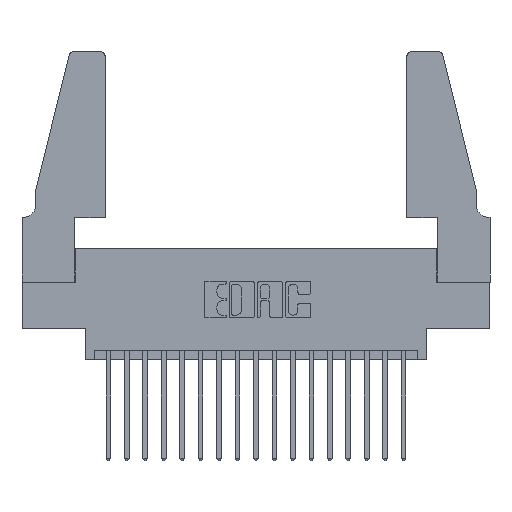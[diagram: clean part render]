
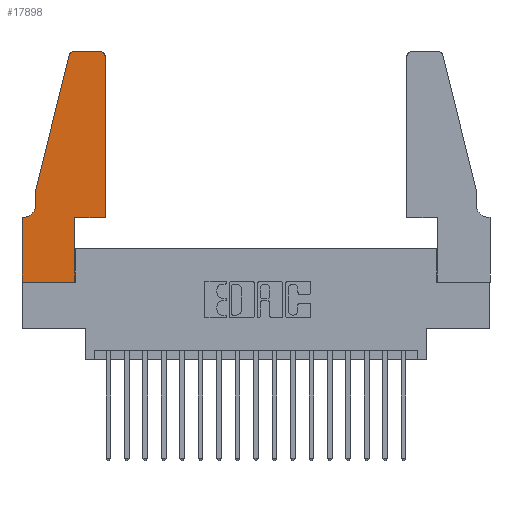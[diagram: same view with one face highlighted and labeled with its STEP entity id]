
A CAD part, top view. The second image highlights one B-rep face of the part: STEP entity #17898.
In plain terms, the highlighted planar face has unit normal (0, 0, 1).
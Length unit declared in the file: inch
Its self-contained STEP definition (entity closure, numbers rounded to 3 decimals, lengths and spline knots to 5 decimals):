
#21 = LINE ( 'NONE', #6034, #14858 ) ;
#507 = CARTESIAN_POINT ( 'NONE',  ( 0., 0., 0.37 ) ) ;
#840 = VERTEX_POINT ( 'NONE', #17186 ) ;
#1100 = DIRECTION ( 'NONE',  ( 0., 0., 1. ) ) ;
#1206 = DIRECTION ( 'NONE',  ( 0., 0., 1. ) ) ;
#1259 = ORIENTED_EDGE ( 'NONE', *, *, #5324, .T. ) ;
#1318 = CIRCLE ( 'NONE', #5021, 0.03 ) ;
#1538 = VECTOR ( 'NONE', #3519, 39.37008 ) ;
#1597 = VECTOR ( 'NONE', #3736, 39.37008 ) ;
#1655 = CARTESIAN_POINT ( 'NONE',  ( 0.4505, 0.35, 0.37 ) ) ;
#1902 = EDGE_CURVE ( 'NONE', #840, #3299, #11785, .T. ) ;
#2050 = EDGE_CURVE ( 'NONE', #11786, #7274, #18245, .T. ) ;
#2129 = CARTESIAN_POINT ( 'NONE',  ( 0.0055, 0.35, 0.37 ) ) ;
#2143 = EDGE_CURVE ( 'NONE', #5489, #8477, #16881, .T. ) ;
#2196 = ORIENTED_EDGE ( 'NONE', *, *, #7530, .T. ) ;
#2276 = CARTESIAN_POINT ( 'NONE',  ( 0.4505, 0.35, 0.37 ) ) ;
#2293 = FACE_OUTER_BOUND ( 'NONE', #11390, .T. ) ;
#3299 = VERTEX_POINT ( 'NONE', #5409 ) ;
#3519 = DIRECTION ( 'NONE',  ( 1., 0., 0. ) ) ;
#3605 = VERTEX_POINT ( 'NONE', #13110 ) ;
#3736 = DIRECTION ( 'NONE',  ( 0., 1., 0. ) ) ;
#3822 = CARTESIAN_POINT ( 'NONE',  ( 0.2865, 0.35, 0.37 ) ) ;
#3868 = VECTOR ( 'NONE', #7863, 39.37008 ) ;
#3891 = CARTESIAN_POINT ( 'NONE',  ( 0.4205, 1.25, 0.37 ) ) ;
#3926 = LINE ( 'NONE', #3822, #7421 ) ;
#4071 = VERTEX_POINT ( 'NONE', #13634 ) ;
#4606 = AXIS2_PLACEMENT_3D ( 'NONE', #5490, #1100, #11475 ) ;
#5021 = AXIS2_PLACEMENT_3D ( 'NONE', #5882, #16181, #7387 ) ;
#5324 = EDGE_CURVE ( 'NONE', #3299, #8935, #12471, .T. ) ;
#5409 = CARTESIAN_POINT ( 'NONE',  ( 0., 0., 0.37 ) ) ;
#5489 = VERTEX_POINT ( 'NONE', #3891 ) ;
#5490 = CARTESIAN_POINT ( 'NONE',  ( 0., 0.35, 0.37 ) ) ;
#5882 = CARTESIAN_POINT ( 'NONE',  ( 0.284, 1.22, 0.37 ) ) ;
#6034 = CARTESIAN_POINT ( 'NONE',  ( 0.0755, 0.5, 0.37 ) ) ;
#6742 = CARTESIAN_POINT ( 'NONE',  ( 0.4505, 0.35, 0.37 ) ) ;
#7274 = VERTEX_POINT ( 'NONE', #2129 ) ;
#7327 = DIRECTION ( 'NONE',  ( 0., -1., 0. ) ) ;
#7387 = DIRECTION ( 'NONE',  ( 1., 0., 0. ) ) ;
#7421 = VECTOR ( 'NONE', #9818, 39.37008 ) ;
#7530 = EDGE_CURVE ( 'NONE', #4071, #5489, #17375, .T. ) ;
#7652 = EDGE_CURVE ( 'NONE', #7274, #840, #15588, .T. ) ;
#7863 = DIRECTION ( 'NONE',  ( -0.239, -0.971, 0. ) ) ;
#7945 = AXIS2_PLACEMENT_3D ( 'NONE', #10101, #1206, #11587 ) ;
#8123 = CARTESIAN_POINT ( 'NONE',  ( 0.2865, 0.35, 0.37 ) ) ;
#8232 = VECTOR ( 'NONE', #10280, 39.37008 ) ;
#8409 = VERTEX_POINT ( 'NONE', #10510 ) ;
#8477 = VERTEX_POINT ( 'NONE', #13635 ) ;
#8532 = EDGE_CURVE ( 'NONE', #8409, #3605, #11319, .T. ) ;
#8621 = ORIENTED_EDGE ( 'NONE', *, *, #17179, .T. ) ;
#8866 = EDGE_CURVE ( 'NONE', #8477, #8409, #1318, .T. ) ;
#8911 = LINE ( 'NONE', #1655, #12887 ) ;
#8935 = VERTEX_POINT ( 'NONE', #14876 ) ;
#9498 = ORIENTED_EDGE ( 'NONE', *, *, #7652, .T. ) ;
#9517 = LINE ( 'NONE', #2276, #1597 ) ;
#9774 = CARTESIAN_POINT ( 'NONE',  ( 0.0055, 0.42, 0.37 ) ) ;
#9818 = DIRECTION ( 'NONE',  ( 0., 1., 0. ) ) ;
#9977 = AXIS2_PLACEMENT_3D ( 'NONE', #9774, #11076, #11170 ) ;
#9987 = PLANE ( 'NONE',  #4606 ) ;
#10101 = CARTESIAN_POINT ( 'NONE',  ( 0.4205, 1.22, 0.37 ) ) ;
#10129 = ORIENTED_EDGE ( 'NONE', *, *, #11989, .T. ) ;
#10280 = DIRECTION ( 'NONE',  ( -1., 0., 0. ) ) ;
#10510 = CARTESIAN_POINT ( 'NONE',  ( 0.25487, 1.22718, 0.37 ) ) ;
#11076 = DIRECTION ( 'NONE',  ( 0., 0., -1. ) ) ;
#11170 = DIRECTION ( 'NONE',  ( -1., 0., 0. ) ) ;
#11319 = LINE ( 'NONE', #18081, #3868 ) ;
#11334 = VECTOR ( 'NONE', #7327, 39.37008 ) ;
#11390 = EDGE_LOOP ( 'NONE', ( #13086, #13402, #16027, #10129, #18684, #9498, #16604, #1259, #8621, #15460, #16996, #2196 ) ) ;
#11475 = DIRECTION ( 'NONE',  ( 1., 0., 0. ) ) ;
#11587 = DIRECTION ( 'NONE',  ( 1., 0., 0. ) ) ;
#11785 = LINE ( 'NONE', #507, #11334 ) ;
#11786 = VERTEX_POINT ( 'NONE', #18594 ) ;
#11989 = EDGE_CURVE ( 'NONE', #3605, #11786, #21, .T. ) ;
#12042 = DIRECTION ( 'NONE',  ( 1., 0., 0. ) ) ;
#12471 = LINE ( 'NONE', #13910, #1538 ) ;
#12887 = VECTOR ( 'NONE', #12042, 39.37008 ) ;
#13086 = ORIENTED_EDGE ( 'NONE', *, *, #2143, .T. ) ;
#13110 = CARTESIAN_POINT ( 'NONE',  ( 0.0755, 0.5, 0.37 ) ) ;
#13402 = ORIENTED_EDGE ( 'NONE', *, *, #8866, .T. ) ;
#13634 = CARTESIAN_POINT ( 'NONE',  ( 0.4505, 1.22, 0.37 ) ) ;
#13635 = CARTESIAN_POINT ( 'NONE',  ( 0.284, 1.25, 0.37 ) ) ;
#13910 = CARTESIAN_POINT ( 'NONE',  ( 0., 0., 0.37 ) ) ;
#14063 = VERTEX_POINT ( 'NONE', #8123 ) ;
#14094 = EDGE_CURVE ( 'NONE', #14117, #4071, #9517, .T. ) ;
#14117 = VERTEX_POINT ( 'NONE', #6742 ) ;
#14733 = CARTESIAN_POINT ( 'NONE',  ( 0.0755, 0.35, 0.37 ) ) ;
#14858 = VECTOR ( 'NONE', #16390, 39.37008 ) ;
#14876 = CARTESIAN_POINT ( 'NONE',  ( 0.2865, 0., 0.37 ) ) ;
#14994 = EDGE_CURVE ( 'NONE', #14063, #14117, #8911, .T. ) ;
#15460 = ORIENTED_EDGE ( 'NONE', *, *, #14994, .T. ) ;
#15588 = LINE ( 'NONE', #14733, #8232 ) ;
#15710 = DIRECTION ( 'NONE',  ( -1., 0., 0. ) ) ;
#16027 = ORIENTED_EDGE ( 'NONE', *, *, #8532, .T. ) ;
#16181 = DIRECTION ( 'NONE',  ( 0., 0., 1. ) ) ;
#16390 = DIRECTION ( 'NONE',  ( 0., -1., 0. ) ) ;
#16431 = VECTOR ( 'NONE', #15710, 39.37008 ) ;
#16604 = ORIENTED_EDGE ( 'NONE', *, *, #1902, .T. ) ;
#16881 = LINE ( 'NONE', #17586, #16431 ) ;
#16996 = ORIENTED_EDGE ( 'NONE', *, *, #14094, .T. ) ;
#17179 = EDGE_CURVE ( 'NONE', #8935, #14063, #3926, .T. ) ;
#17186 = CARTESIAN_POINT ( 'NONE',  ( 0., 0.35, 0.37 ) ) ;
#17375 = CIRCLE ( 'NONE', #7945, 0.03 ) ;
#17586 = CARTESIAN_POINT ( 'NONE',  ( 0.2605, 1.25, 0.37 ) ) ;
#17898 = ADVANCED_FACE ( 'NONE', ( #2293 ), #9987, .T. ) ;
#18081 = CARTESIAN_POINT ( 'NONE',  ( 0.0755, 0.5, 0.37 ) ) ;
#18245 = CIRCLE ( 'NONE', #9977, 0.07 ) ;
#18594 = CARTESIAN_POINT ( 'NONE',  ( 0.0755, 0.42, 0.37 ) ) ;
#18684 = ORIENTED_EDGE ( 'NONE', *, *, #2050, .T. ) ;
